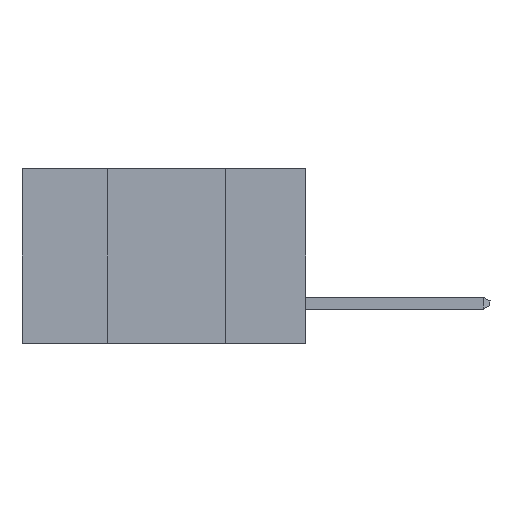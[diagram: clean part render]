
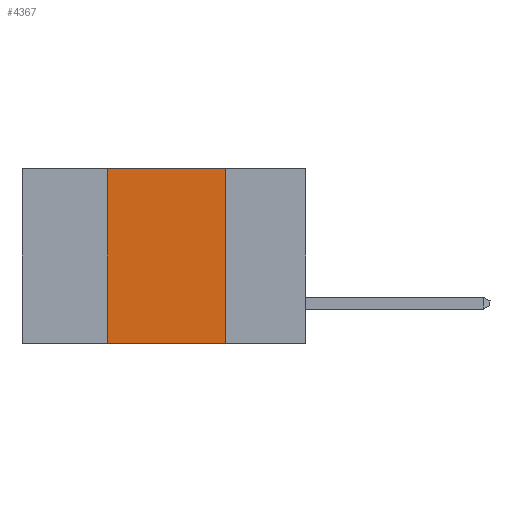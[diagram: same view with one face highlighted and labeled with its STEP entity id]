
A CAD part, left-side view. The second image highlights one B-rep face of the part: STEP entity #4367.
In plain terms, the highlighted planar face has unit normal (-1, 0, 0).
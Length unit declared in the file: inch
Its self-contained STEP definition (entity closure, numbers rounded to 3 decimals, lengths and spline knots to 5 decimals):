
#389 = PLANE ( 'NONE',  #2898 ) ;
#608 = EDGE_CURVE ( 'NONE', #1725, #7540, #1152, .T. ) ;
#712 = VECTOR ( 'NONE', #11750, 39.37008 ) ;
#875 = CARTESIAN_POINT ( 'NONE',  ( 0., 0.17, 0. ) ) ;
#1152 = LINE ( 'NONE', #7350, #10980 ) ;
#1278 = DIRECTION ( 'NONE',  ( 0., -1., 0. ) ) ;
#1499 = CARTESIAN_POINT ( 'NONE',  ( 0., 0.42, 0. ) ) ;
#1639 = CARTESIAN_POINT ( 'NONE',  ( 0., 0.42, -0.37 ) ) ;
#1725 = VERTEX_POINT ( 'NONE', #12644 ) ;
#1807 = VECTOR ( 'NONE', #2200, 39.37008 ) ;
#1813 = EDGE_CURVE ( 'NONE', #6609, #4197, #11024, .T. ) ;
#2032 = EDGE_LOOP ( 'NONE', ( #5374, #9189, #8298, #3556 ) ) ;
#2200 = DIRECTION ( 'NONE',  ( 0., 0., -1. ) ) ;
#2554 = DIRECTION ( 'NONE',  ( 1., 0., 0. ) ) ;
#2898 = AXIS2_PLACEMENT_3D ( 'NONE', #4521, #2554, #7524 ) ;
#3556 = ORIENTED_EDGE ( 'NONE', *, *, #608, .T. ) ;
#3635 = EDGE_CURVE ( 'NONE', #4197, #7540, #11282, .T. ) ;
#4197 = VERTEX_POINT ( 'NONE', #875 ) ;
#4367 = ADVANCED_FACE ( 'NONE', ( #7590 ), #389, .F. ) ;
#4521 = CARTESIAN_POINT ( 'NONE',  ( 0., 0.6, 0. ) ) ;
#5374 = ORIENTED_EDGE ( 'NONE', *, *, #3635, .F. ) ;
#6580 = CARTESIAN_POINT ( 'NONE',  ( 0., 0.17, -0.37 ) ) ;
#6609 = VERTEX_POINT ( 'NONE', #1499 ) ;
#7350 = CARTESIAN_POINT ( 'NONE',  ( 0., 0.6, -0.37 ) ) ;
#7524 = DIRECTION ( 'NONE',  ( 0., 0., -1. ) ) ;
#7540 = VERTEX_POINT ( 'NONE', #6580 ) ;
#7590 = FACE_OUTER_BOUND ( 'NONE', #2032, .T. ) ;
#8187 = VECTOR ( 'NONE', #10966, 39.37008 ) ;
#8298 = ORIENTED_EDGE ( 'NONE', *, *, #12741, .F. ) ;
#8367 = CARTESIAN_POINT ( 'NONE',  ( 0., 0.17, -0.37 ) ) ;
#8705 = LINE ( 'NONE', #1639, #712 ) ;
#9189 = ORIENTED_EDGE ( 'NONE', *, *, #1813, .F. ) ;
#9948 = CARTESIAN_POINT ( 'NONE',  ( 0., 0.6, 0. ) ) ;
#10966 = DIRECTION ( 'NONE',  ( 0., -1., 0. ) ) ;
#10980 = VECTOR ( 'NONE', #1278, 39.37008 ) ;
#11024 = LINE ( 'NONE', #9948, #8187 ) ;
#11282 = LINE ( 'NONE', #8367, #1807 ) ;
#11750 = DIRECTION ( 'NONE',  ( 0., 0., 1. ) ) ;
#12644 = CARTESIAN_POINT ( 'NONE',  ( 0., 0.42, -0.37 ) ) ;
#12741 = EDGE_CURVE ( 'NONE', #1725, #6609, #8705, .T. ) ;
